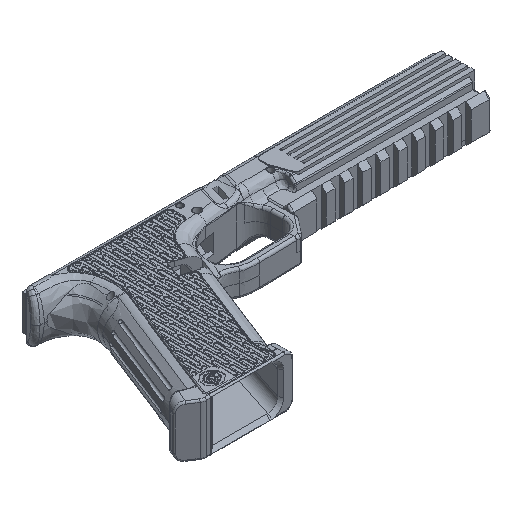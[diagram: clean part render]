
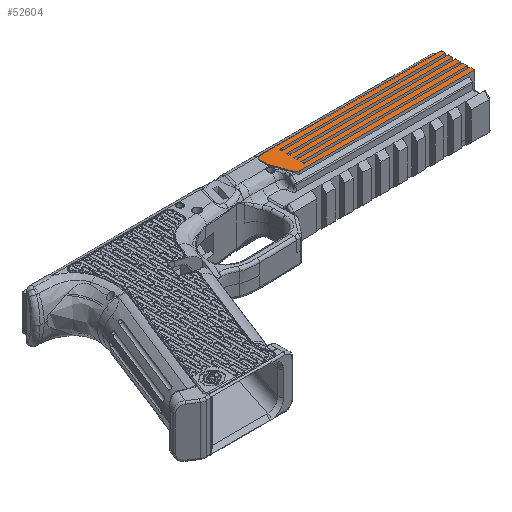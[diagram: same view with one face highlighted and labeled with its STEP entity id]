
A CAD part, isometric view. The second image highlights one B-rep face of the part: STEP entity #52604.
In plain terms, the highlighted planar face has unit normal (0, 0, 1).
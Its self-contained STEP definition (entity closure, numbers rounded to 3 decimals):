
#5085=PLANE('',#55685);
#6287=FACE_OUTER_BOUND('',#9323,.T.);
#9323=EDGE_LOOP('',(#35840,#35841,#35842,#35843,#35844,#35845,#35846,#35847,
#35848,#35849,#35850,#35851,#35852,#35853,#35854,#35855,#35856,#35857,#35858,
#35859,#35860,#35861,#35862,#35863));
#12470=LINE('',#66873,#16875);
#12479=LINE('',#66896,#16884);
#12493=LINE('',#66933,#16898);
#12507=LINE('',#66970,#16912);
#12508=LINE('',#66973,#16913);
#12515=LINE('',#66988,#16920);
#12517=LINE('',#66994,#16922);
#12521=LINE('',#67004,#16926);
#12554=LINE('',#67544,#16959);
#12555=LINE('',#67548,#16960);
#12556=LINE('',#67552,#16961);
#12557=LINE('',#67553,#16962);
#12558=LINE('',#67555,#16963);
#12559=LINE('',#67557,#16964);
#12560=LINE('',#67558,#16965);
#12561=LINE('',#67559,#16966);
#12562=LINE('',#67561,#16967);
#12563=LINE('',#67562,#16968);
#12564=LINE('',#67564,#16969);
#12565=LINE('',#67566,#16970);
#12566=LINE('',#67567,#16971);
#16875=VECTOR('',#57913,10.);
#16884=VECTOR('',#57932,10.);
#16898=VECTOR('',#57958,10.);
#16912=VECTOR('',#57988,10.);
#16913=VECTOR('',#57991,10.);
#16920=VECTOR('',#58002,10.);
#16922=VECTOR('',#58008,10.);
#16926=VECTOR('',#58018,10.);
#16959=VECTOR('',#58119,10.);
#16960=VECTOR('',#58122,10.);
#16961=VECTOR('',#58125,10.);
#16962=VECTOR('',#58126,10.);
#16963=VECTOR('',#58127,10.);
#16964=VECTOR('',#58128,10.);
#16965=VECTOR('',#58129,10.);
#16966=VECTOR('',#58130,10.);
#16967=VECTOR('',#58131,10.);
#16968=VECTOR('',#58132,10.);
#16969=VECTOR('',#58133,10.);
#16970=VECTOR('',#58134,10.);
#16971=VECTOR('',#58135,10.);
#21295=CIRCLE('',#55683,2.);
#21297=CIRCLE('',#55686,2.);
#21298=CIRCLE('',#55687,2.);
#21896=VERTEX_POINT('',#66870);
#21897=VERTEX_POINT('',#66872);
#21905=VERTEX_POINT('',#66893);
#21906=VERTEX_POINT('',#66895);
#21922=VERTEX_POINT('',#66930);
#21923=VERTEX_POINT('',#66932);
#21936=VERTEX_POINT('',#66964);
#21938=VERTEX_POINT('',#66968);
#21939=VERTEX_POINT('',#66972);
#21945=VERTEX_POINT('',#66986);
#21947=VERTEX_POINT('',#66991);
#21950=VERTEX_POINT('',#67002);
#22008=VERTEX_POINT('',#67534);
#22009=VERTEX_POINT('',#67535);
#22012=VERTEX_POINT('',#67543);
#22013=VERTEX_POINT('',#67545);
#22014=VERTEX_POINT('',#67547);
#22015=VERTEX_POINT('',#67549);
#22016=VERTEX_POINT('',#67551);
#22017=VERTEX_POINT('',#67554);
#22018=VERTEX_POINT('',#67556);
#22019=VERTEX_POINT('',#67560);
#22020=VERTEX_POINT('',#67563);
#22021=VERTEX_POINT('',#67565);
#27313=EDGE_CURVE('',#21896,#21897,#12470,.T.);
#27324=EDGE_CURVE('',#21905,#21906,#12479,.T.);
#27342=EDGE_CURVE('',#21922,#21923,#12493,.T.);
#27360=EDGE_CURVE('',#21938,#21936,#12507,.T.);
#27361=EDGE_CURVE('',#21936,#21939,#12508,.T.);
#27369=EDGE_CURVE('',#21945,#21922,#12515,.T.);
#27372=EDGE_CURVE('',#21906,#21947,#12517,.T.);
#27377=EDGE_CURVE('',#21950,#21896,#12521,.T.);
#27453=EDGE_CURVE('',#22008,#22009,#21295,.T.);
#27457=EDGE_CURVE('',#22012,#22008,#12554,.T.);
#27458=EDGE_CURVE('',#22012,#22013,#21297,.T.);
#27459=EDGE_CURVE('',#22014,#22013,#12555,.T.);
#27460=EDGE_CURVE('',#22014,#22015,#21298,.T.);
#27461=EDGE_CURVE('',#22016,#22015,#12556,.F.);
#27462=EDGE_CURVE('',#21897,#22016,#12557,.T.);
#27463=EDGE_CURVE('',#22017,#21950,#12558,.T.);
#27464=EDGE_CURVE('',#22018,#22017,#12559,.T.);
#27465=EDGE_CURVE('',#21947,#22018,#12560,.T.);
#27466=EDGE_CURVE('',#21923,#21905,#12561,.T.);
#27467=EDGE_CURVE('',#22019,#21945,#12562,.T.);
#27468=EDGE_CURVE('',#21939,#22019,#12563,.T.);
#27469=EDGE_CURVE('',#22020,#21938,#12564,.T.);
#27470=EDGE_CURVE('',#22021,#22020,#12565,.T.);
#27471=EDGE_CURVE('',#22009,#22021,#12566,.T.);
#35840=ORIENTED_EDGE('',*,*,#27453,.F.);
#35841=ORIENTED_EDGE('',*,*,#27457,.F.);
#35842=ORIENTED_EDGE('',*,*,#27458,.T.);
#35843=ORIENTED_EDGE('',*,*,#27459,.F.);
#35844=ORIENTED_EDGE('',*,*,#27460,.T.);
#35845=ORIENTED_EDGE('',*,*,#27461,.F.);
#35846=ORIENTED_EDGE('',*,*,#27462,.F.);
#35847=ORIENTED_EDGE('',*,*,#27313,.F.);
#35848=ORIENTED_EDGE('',*,*,#27377,.F.);
#35849=ORIENTED_EDGE('',*,*,#27463,.F.);
#35850=ORIENTED_EDGE('',*,*,#27464,.F.);
#35851=ORIENTED_EDGE('',*,*,#27465,.F.);
#35852=ORIENTED_EDGE('',*,*,#27372,.F.);
#35853=ORIENTED_EDGE('',*,*,#27324,.F.);
#35854=ORIENTED_EDGE('',*,*,#27466,.F.);
#35855=ORIENTED_EDGE('',*,*,#27342,.F.);
#35856=ORIENTED_EDGE('',*,*,#27369,.F.);
#35857=ORIENTED_EDGE('',*,*,#27467,.F.);
#35858=ORIENTED_EDGE('',*,*,#27468,.F.);
#35859=ORIENTED_EDGE('',*,*,#27361,.F.);
#35860=ORIENTED_EDGE('',*,*,#27360,.F.);
#35861=ORIENTED_EDGE('',*,*,#27469,.F.);
#35862=ORIENTED_EDGE('',*,*,#27470,.F.);
#35863=ORIENTED_EDGE('',*,*,#27471,.F.);
#52604=ADVANCED_FACE('',(#6287),#5085,.F.);
#55683=AXIS2_PLACEMENT_3D('',#67536,#58111,#58112);
#55685=AXIS2_PLACEMENT_3D('',#67542,#58117,#58118);
#55686=AXIS2_PLACEMENT_3D('',#67546,#58120,#58121);
#55687=AXIS2_PLACEMENT_3D('',#67550,#58123,#58124);
#57913=DIRECTION('',(1.,0.001,0.));
#57932=DIRECTION('',(-1.,-0.001,0.));
#57958=DIRECTION('',(1.,0.001,0.));
#57988=DIRECTION('',(0.001,-1.,0.));
#57991=DIRECTION('',(1.,0.001,0.));
#58002=DIRECTION('',(0.001,-1.,0.));
#58008=DIRECTION('',(0.001,-1.,0.));
#58018=DIRECTION('',(0.001,-1.,0.));
#58111=DIRECTION('center_axis',(0.,0.,
-1.));
#58112=DIRECTION('ref_axis',(-0.707,0.707,0.));
#58117=DIRECTION('center_axis',(0.,0.,
-1.));
#58118=DIRECTION('ref_axis',(-1.,0.,0.));
#58119=DIRECTION('',(0.,1.,0.));
#58120=DIRECTION('center_axis',(0.,0.,
1.));
#58121=DIRECTION('ref_axis',(-0.985,-0.174,0.));
#58122=DIRECTION('',(-0.343,0.939,0.));
#58123=DIRECTION('center_axis',(0.,0.,
1.));
#58124=DIRECTION('ref_axis',(-0.573,-0.819,0.));
#58125=DIRECTION('',(1.,0.,0.));
#58126=DIRECTION('',(0.,-1.,0.));
#58127=DIRECTION('',(-1.,-0.001,0.));
#58128=DIRECTION('',(0.,-1.,0.));
#58129=DIRECTION('',(1.,0.001,0.));
#58130=DIRECTION('',(0.,-1.,0.));
#58131=DIRECTION('',(-1.,-0.001,0.));
#58132=DIRECTION('',(0.,-1.,0.));
#58133=DIRECTION('',(-1.,-0.001,0.));
#58134=DIRECTION('',(0.,-1.,0.));
#58135=DIRECTION('',(1.,0.,0.));
#66870=CARTESIAN_POINT('',(133.919,-20.005,14.853));
#66872=CARTESIAN_POINT('',(225.918,-19.954,14.853));
#66873=CARTESIAN_POINT('',(199.888,-19.969,14.853));
#66893=CARTESIAN_POINT('',(225.918,-14.454,14.853));
#66895=CARTESIAN_POINT('',(133.918,-14.505,14.853));
#66896=CARTESIAN_POINT('',(198.887,-14.469,14.853));
#66930=CARTESIAN_POINT('',(133.919,-12.005,14.853));
#66932=CARTESIAN_POINT('',(225.918,-11.954,14.853));
#66933=CARTESIAN_POINT('',(199.886,-11.969,14.853));
#66964=CARTESIAN_POINT('',(133.919,-8.005,14.853));
#66968=CARTESIAN_POINT('',(133.918,-6.505,14.853));
#66970=CARTESIAN_POINT('',(133.92,-10.348,14.853));
#66972=CARTESIAN_POINT('',(225.918,-7.954,14.853));
#66973=CARTESIAN_POINT('',(199.885,-7.969,14.853));
#66986=CARTESIAN_POINT('',(133.918,-10.505,14.853));
#66988=CARTESIAN_POINT('',(133.919,-12.348,14.853));
#66991=CARTESIAN_POINT('',(133.919,-16.005,14.853));
#66994=CARTESIAN_POINT('',(133.918,-14.348,14.853));
#67002=CARTESIAN_POINT('',(133.918,-18.505,14.853));
#67004=CARTESIAN_POINT('',(133.917,-16.348,14.853));
#67534=CARTESIAN_POINT('',(123.793,-5.955,14.853));
#67535=CARTESIAN_POINT('',(125.793,-3.955,14.853));
#67536=CARTESIAN_POINT('Origin',(125.793,-5.955,14.853));
#67542=CARTESIAN_POINT('Origin',(173.856,-14.168,14.853));
#67543=CARTESIAN_POINT('',(123.793,-10.5,14.853));
#67544=CARTESIAN_POINT('',(123.793,-10.854,14.853));
#67545=CARTESIAN_POINT('',(123.914,-11.186,14.853));
#67546=CARTESIAN_POINT('Origin',(125.793,-10.5,14.853));
#67547=CARTESIAN_POINT('',(127.563,-21.191,14.853));
#67548=CARTESIAN_POINT('',(128.26,-23.102,14.853));
#67549=CARTESIAN_POINT('',(129.442,-22.506,14.853));
#67550=CARTESIAN_POINT('Origin',(129.442,-20.506,14.853));
#67551=CARTESIAN_POINT('',(225.918,-22.506,14.853));
#67552=CARTESIAN_POINT('',(198.887,-22.506,14.853));
#67553=CARTESIAN_POINT('',(225.918,-17.824,14.853));
#67554=CARTESIAN_POINT('',(225.918,-18.454,14.853));
#67555=CARTESIAN_POINT('',(198.888,-18.469,14.853));
#67556=CARTESIAN_POINT('',(225.918,-15.954,14.853));
#67557=CARTESIAN_POINT('',(225.918,-10.312,14.853));
#67558=CARTESIAN_POINT('',(199.887,-15.969,14.853));
#67559=CARTESIAN_POINT('',(225.918,-10.312,14.853));
#67560=CARTESIAN_POINT('',(225.918,-10.454,14.853));
#67561=CARTESIAN_POINT('',(198.886,-10.469,14.853));
#67562=CARTESIAN_POINT('',(225.918,-10.312,14.853));
#67563=CARTESIAN_POINT('',(225.918,-6.454,14.853));
#67564=CARTESIAN_POINT('',(198.885,-6.469,14.853));
#67565=CARTESIAN_POINT('',(225.918,-3.955,14.853));
#67566=CARTESIAN_POINT('',(225.918,-9.811,14.853));
#67567=CARTESIAN_POINT('',(148.824,-3.955,14.853));
